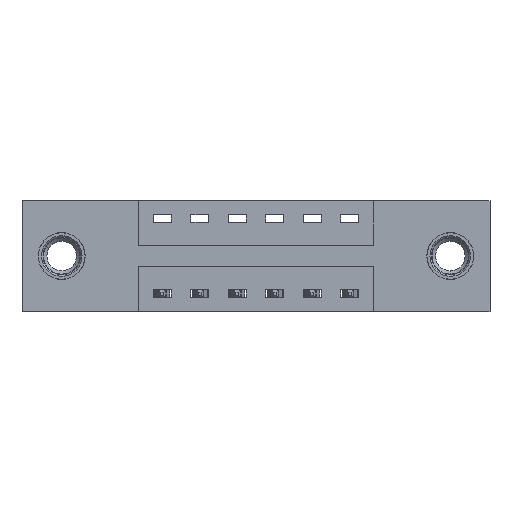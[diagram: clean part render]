
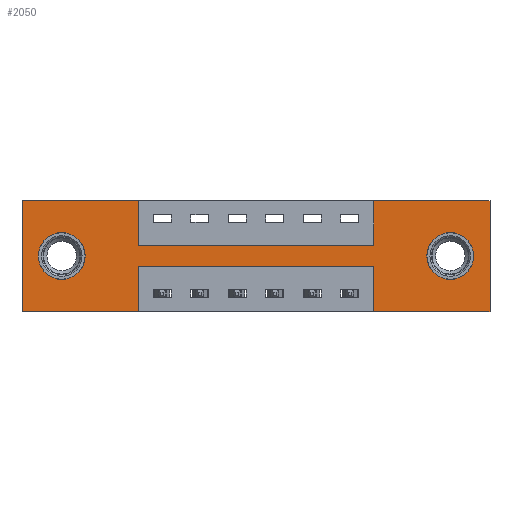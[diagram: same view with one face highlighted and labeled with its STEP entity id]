
A CAD part, front view. The second image highlights one B-rep face of the part: STEP entity #2050.
In plain terms, the highlighted planar face has unit normal (0, -1, 0).
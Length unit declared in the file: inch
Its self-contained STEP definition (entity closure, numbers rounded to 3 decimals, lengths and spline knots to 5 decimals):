
#157 = DIRECTION ( 'NONE',  ( 0., 1., 0. ) ) ;
#162 = EDGE_CURVE ( 'NONE', #3270, #4690, #4498, .T. ) ;
#176 = EDGE_CURVE ( 'NONE', #1032, #8727, #2475, .T. ) ;
#267 = CARTESIAN_POINT ( 'NONE',  ( 0., 0., 0. ) ) ;
#325 = CARTESIAN_POINT ( 'NONE',  ( 0., 0., -0.37 ) ) ;
#433 = CARTESIAN_POINT ( 'NONE',  ( 0.1325, 0., -0.107 ) ) ;
#434 = CARTESIAN_POINT ( 'NONE',  ( 0., 0., -0.37 ) ) ;
#735 = EDGE_CURVE ( 'NONE', #6157, #7298, #7558, .T. ) ;
#879 = FACE_BOUND ( 'NONE', #8972, .T. ) ;
#891 = DIRECTION ( 'NONE',  ( 0., 0., 1. ) ) ;
#934 = VERTEX_POINT ( 'NONE', #8304 ) ;
#1032 = VERTEX_POINT ( 'NONE', #6153 ) ;
#1255 = LINE ( 'NONE', #3962, #7057 ) ;
#1256 = CARTESIAN_POINT ( 'NONE',  ( 1.4275, 0., -0.107 ) ) ;
#1264 = VERTEX_POINT ( 'NONE', #267 ) ;
#1445 = VECTOR ( 'NONE', #8272, 39.37008 ) ;
#1744 = EDGE_CURVE ( 'NONE', #2864, #5604, #1255, .T. ) ;
#1772 = CARTESIAN_POINT ( 'NONE',  ( 0., 0., -0.37 ) ) ;
#1856 = DIRECTION ( 'NONE',  ( -1., 0., 0. ) ) ;
#1963 = DIRECTION ( 'NONE',  ( 0., 1., 0. ) ) ;
#2037 = CARTESIAN_POINT ( 'NONE',  ( 0., 0., 0. ) ) ;
#2050 = ADVANCED_FACE ( 'NONE', ( #879, #4699, #2682 ), #6527, .T. ) ;
#2054 = ORIENTED_EDGE ( 'NONE', *, *, #5250, .F. ) ;
#2081 = EDGE_CURVE ( 'NONE', #5604, #7106, #6217, .T. ) ;
#2188 = CIRCLE ( 'NONE', #2938, 0.078 ) ;
#2294 = VECTOR ( 'NONE', #5190, 39.37008 ) ;
#2345 = CARTESIAN_POINT ( 'NONE',  ( 1.1725, 0., 0. ) ) ;
#2467 = EDGE_CURVE ( 'NONE', #7961, #6157, #4218, .T. ) ;
#2475 = LINE ( 'NONE', #434, #8278 ) ;
#2479 = CARTESIAN_POINT ( 'NONE',  ( 1.4275, 0., -0.185 ) ) ;
#2481 = EDGE_CURVE ( 'NONE', #5618, #8293, #2188, .T. ) ;
#2485 = ORIENTED_EDGE ( 'NONE', *, *, #2467, .F. ) ;
#2509 = CARTESIAN_POINT ( 'NONE',  ( 1.1725, 0., -0.37 ) ) ;
#2682 = FACE_OUTER_BOUND ( 'NONE', #5941, .T. ) ;
#2743 = ORIENTED_EDGE ( 'NONE', *, *, #7792, .F. ) ;
#2744 = LINE ( 'NONE', #2037, #4290 ) ;
#2802 = DIRECTION ( 'NONE',  ( 1., 0., 0. ) ) ;
#2857 = DIRECTION ( 'NONE',  ( 0., 1., 0. ) ) ;
#2864 = VERTEX_POINT ( 'NONE', #9087 ) ;
#2879 = ORIENTED_EDGE ( 'NONE', *, *, #8395, .T. ) ;
#2921 = CARTESIAN_POINT ( 'NONE',  ( 1.4275, 0., -0.263 ) ) ;
#2938 = AXIS2_PLACEMENT_3D ( 'NONE', #4728, #157, #5484 ) ;
#3250 = DIRECTION ( 'NONE',  ( 0., 0., -1. ) ) ;
#3270 = VERTEX_POINT ( 'NONE', #1256 ) ;
#3280 = CARTESIAN_POINT ( 'NONE',  ( 1.1725, 0., -0.22 ) ) ;
#3360 = CARTESIAN_POINT ( 'NONE',  ( 0.3875, 0., -0.15 ) ) ;
#3446 = EDGE_CURVE ( 'NONE', #7298, #1032, #5496, .T. ) ;
#3450 = LINE ( 'NONE', #8375, #5225 ) ;
#3504 = ORIENTED_EDGE ( 'NONE', *, *, #8672, .T. ) ;
#3530 = CARTESIAN_POINT ( 'NONE',  ( 0., 0., -0.37 ) ) ;
#3539 = EDGE_CURVE ( 'NONE', #1264, #2864, #6776, .T. ) ;
#3962 = CARTESIAN_POINT ( 'NONE',  ( 0.3875, 0., 0. ) ) ;
#4127 = DIRECTION ( 'NONE',  ( 0., 0., 1. ) ) ;
#4162 = AXIS2_PLACEMENT_3D ( 'NONE', #3530, #4300, #9548 ) ;
#4218 = LINE ( 'NONE', #6199, #4687 ) ;
#4229 = VECTOR ( 'NONE', #5840, 39.37008 ) ;
#4261 = CIRCLE ( 'NONE', #5776, 0.078 ) ;
#4290 = VECTOR ( 'NONE', #2802, 39.37008 ) ;
#4300 = DIRECTION ( 'NONE',  ( 0., -1., 0. ) ) ;
#4378 = ORIENTED_EDGE ( 'NONE', *, *, #2481, .T. ) ;
#4498 = CIRCLE ( 'NONE', #9019, 0.078 ) ;
#4598 = DIRECTION ( 'NONE',  ( 0., 0., 1. ) ) ;
#4687 = VECTOR ( 'NONE', #891, 39.37008 ) ;
#4690 = VERTEX_POINT ( 'NONE', #2921 ) ;
#4699 = FACE_BOUND ( 'NONE', #9046, .T. ) ;
#4728 = CARTESIAN_POINT ( 'NONE',  ( 0.1325, 0., -0.185 ) ) ;
#4786 = CARTESIAN_POINT ( 'NONE',  ( 0.3875, 0., -0.22 ) ) ;
#4847 = ORIENTED_EDGE ( 'NONE', *, *, #735, .F. ) ;
#4993 = CARTESIAN_POINT ( 'NONE',  ( 0.3875, 0., -0.22 ) ) ;
#5190 = DIRECTION ( 'NONE',  ( 0., 0., -1. ) ) ;
#5225 = VECTOR ( 'NONE', #4598, 39.37008 ) ;
#5250 = EDGE_CURVE ( 'NONE', #9755, #934, #6313, .T. ) ;
#5366 = CARTESIAN_POINT ( 'NONE',  ( 0., 0., 0. ) ) ;
#5484 = DIRECTION ( 'NONE',  ( 0., 0., 1. ) ) ;
#5496 = LINE ( 'NONE', #9007, #1445 ) ;
#5553 = VECTOR ( 'NONE', #9504, 39.37008 ) ;
#5604 = VERTEX_POINT ( 'NONE', #3360 ) ;
#5618 = VERTEX_POINT ( 'NONE', #9376 ) ;
#5664 = CIRCLE ( 'NONE', #9104, 0.078 ) ;
#5676 = VECTOR ( 'NONE', #4127, 39.37008 ) ;
#5742 = DIRECTION ( 'NONE',  ( -1., 0., 0. ) ) ;
#5776 = AXIS2_PLACEMENT_3D ( 'NONE', #7384, #2857, #8152 ) ;
#5797 = CARTESIAN_POINT ( 'NONE',  ( 1.56, 0., 0. ) ) ;
#5840 = DIRECTION ( 'NONE',  ( 1., 0., 0. ) ) ;
#5941 = EDGE_LOOP ( 'NONE', ( #6703, #4847, #2485, #7365, #2054, #6893, #2743, #9350, #6385, #7653, #8236, #7534 ) ) ;
#6120 = DIRECTION ( 'NONE',  ( 1., 0., 0. ) ) ;
#6153 = CARTESIAN_POINT ( 'NONE',  ( 0.3875, 0., -0.37 ) ) ;
#6157 = VERTEX_POINT ( 'NONE', #3280 ) ;
#6199 = CARTESIAN_POINT ( 'NONE',  ( 1.1725, 0., -0.37 ) ) ;
#6217 = LINE ( 'NONE', #7323, #4229 ) ;
#6306 = VECTOR ( 'NONE', #6120, 39.37008 ) ;
#6313 = LINE ( 'NONE', #5797, #2294 ) ;
#6385 = ORIENTED_EDGE ( 'NONE', *, *, #1744, .F. ) ;
#6490 = CARTESIAN_POINT ( 'NONE',  ( 1.4275, 0., -0.185 ) ) ;
#6527 = PLANE ( 'NONE',  #4162 ) ;
#6703 = ORIENTED_EDGE ( 'NONE', *, *, #3446, .F. ) ;
#6776 = LINE ( 'NONE', #5366, #6306 ) ;
#6854 = CARTESIAN_POINT ( 'NONE',  ( 1.56, 0., 0. ) ) ;
#6862 = EDGE_CURVE ( 'NONE', #934, #7961, #9463, .T. ) ;
#6893 = ORIENTED_EDGE ( 'NONE', *, *, #6999, .F. ) ;
#6926 = DIRECTION ( 'NONE',  ( 0., 0., -1. ) ) ;
#6999 = EDGE_CURVE ( 'NONE', #7817, #9755, #2744, .T. ) ;
#7057 = VECTOR ( 'NONE', #6926, 39.37008 ) ;
#7106 = VERTEX_POINT ( 'NONE', #7554 ) ;
#7148 = CARTESIAN_POINT ( 'NONE',  ( 0., 0., 0. ) ) ;
#7259 = DIRECTION ( 'NONE',  ( 0., 0., -1. ) ) ;
#7298 = VERTEX_POINT ( 'NONE', #4786 ) ;
#7323 = CARTESIAN_POINT ( 'NONE',  ( 0.3875, 0., -0.15 ) ) ;
#7365 = ORIENTED_EDGE ( 'NONE', *, *, #6862, .F. ) ;
#7384 = CARTESIAN_POINT ( 'NONE',  ( 0.1325, 0., -0.185 ) ) ;
#7468 = VECTOR ( 'NONE', #1856, 39.37008 ) ;
#7534 = ORIENTED_EDGE ( 'NONE', *, *, #176, .F. ) ;
#7554 = CARTESIAN_POINT ( 'NONE',  ( 1.1725, 0., -0.15 ) ) ;
#7558 = LINE ( 'NONE', #4993, #5553 ) ;
#7653 = ORIENTED_EDGE ( 'NONE', *, *, #3539, .F. ) ;
#7683 = LINE ( 'NONE', #7148, #5676 ) ;
#7782 = DIRECTION ( 'NONE',  ( 0., 1., 0. ) ) ;
#7792 = EDGE_CURVE ( 'NONE', #7106, #7817, #3450, .T. ) ;
#7817 = VERTEX_POINT ( 'NONE', #2345 ) ;
#7961 = VERTEX_POINT ( 'NONE', #2509 ) ;
#8152 = DIRECTION ( 'NONE',  ( 0., 0., 1. ) ) ;
#8211 = EDGE_CURVE ( 'NONE', #8727, #1264, #7683, .T. ) ;
#8236 = ORIENTED_EDGE ( 'NONE', *, *, #8211, .F. ) ;
#8272 = DIRECTION ( 'NONE',  ( 0., 0., -1. ) ) ;
#8278 = VECTOR ( 'NONE', #5742, 39.37008 ) ;
#8293 = VERTEX_POINT ( 'NONE', #433 ) ;
#8304 = CARTESIAN_POINT ( 'NONE',  ( 1.56, 0., -0.37 ) ) ;
#8375 = CARTESIAN_POINT ( 'NONE',  ( 1.1725, 0., 0. ) ) ;
#8395 = EDGE_CURVE ( 'NONE', #8293, #5618, #4261, .T. ) ;
#8672 = EDGE_CURVE ( 'NONE', #4690, #3270, #5664, .T. ) ;
#8727 = VERTEX_POINT ( 'NONE', #1772 ) ;
#8972 = EDGE_LOOP ( 'NONE', ( #9222, #3504 ) ) ;
#9007 = CARTESIAN_POINT ( 'NONE',  ( 0.3875, 0., -0.37 ) ) ;
#9019 = AXIS2_PLACEMENT_3D ( 'NONE', #6490, #1963, #7259 ) ;
#9046 = EDGE_LOOP ( 'NONE', ( #2879, #4378 ) ) ;
#9087 = CARTESIAN_POINT ( 'NONE',  ( 0.3875, 0., 0. ) ) ;
#9104 = AXIS2_PLACEMENT_3D ( 'NONE', #2479, #7782, #3250 ) ;
#9222 = ORIENTED_EDGE ( 'NONE', *, *, #162, .T. ) ;
#9350 = ORIENTED_EDGE ( 'NONE', *, *, #2081, .F. ) ;
#9376 = CARTESIAN_POINT ( 'NONE',  ( 0.1325, 0., -0.263 ) ) ;
#9463 = LINE ( 'NONE', #325, #7468 ) ;
#9504 = DIRECTION ( 'NONE',  ( -1., 0., 0. ) ) ;
#9548 = DIRECTION ( 'NONE',  ( 0., 0., -1. ) ) ;
#9755 = VERTEX_POINT ( 'NONE', #6854 ) ;
